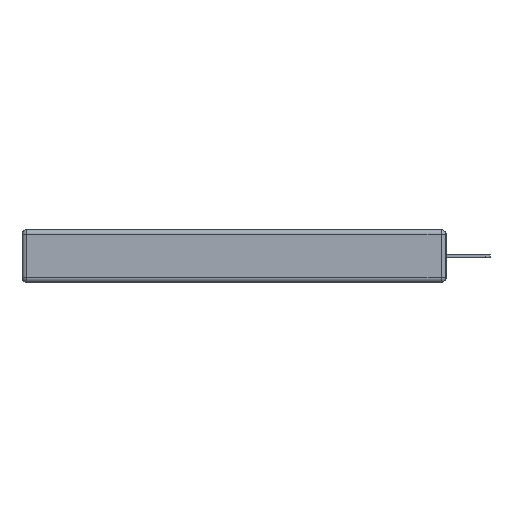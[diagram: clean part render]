
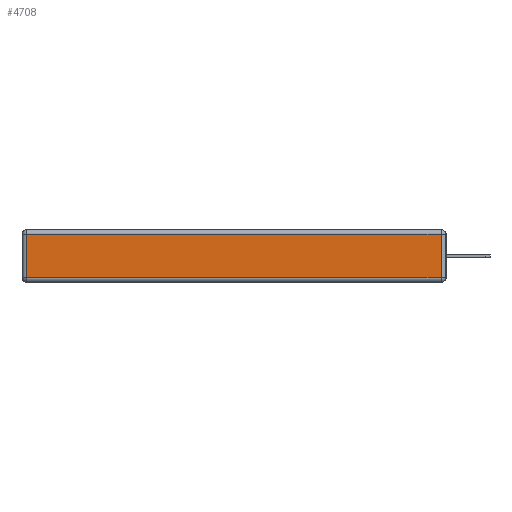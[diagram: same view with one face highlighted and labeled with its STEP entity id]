
A CAD part, left-side view. The second image highlights one B-rep face of the part: STEP entity #4708.
In plain terms, the highlighted planar face has unit normal (-1, 0, 0).
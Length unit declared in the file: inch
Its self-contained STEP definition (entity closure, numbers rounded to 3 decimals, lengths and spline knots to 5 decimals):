
#834 = CARTESIAN_POINT ( 'NONE',  ( 0., 2.72, -0.03 ) ) ;
#927 = EDGE_CURVE ( 'NONE', #22604, #4115, #10498, .T. ) ;
#2394 = CARTESIAN_POINT ( 'NONE',  ( 0., 0., -0.313 ) ) ;
#2729 = VERTEX_POINT ( 'NONE', #834 ) ;
#2935 = VECTOR ( 'NONE', #6644, 39.37008 ) ;
#2946 = CARTESIAN_POINT ( 'NONE',  ( 0., 2.72, -0.313 ) ) ;
#4115 = VERTEX_POINT ( 'NONE', #21625 ) ;
#4242 = EDGE_CURVE ( 'NONE', #6738, #22604, #4624, .T. ) ;
#4624 = LINE ( 'NONE', #2394, #20329 ) ;
#4708 = ADVANCED_FACE ( 'NONE', ( #14742 ), #17619, .T. ) ;
#6498 = ORIENTED_EDGE ( 'NONE', *, *, #17377, .T. ) ;
#6644 = DIRECTION ( 'NONE',  ( 0., 1., 0. ) ) ;
#6738 = VERTEX_POINT ( 'NONE', #2946 ) ;
#6924 = VECTOR ( 'NONE', #21219, 39.37008 ) ;
#7424 = ORIENTED_EDGE ( 'NONE', *, *, #927, .T. ) ;
#8707 = DIRECTION ( 'NONE',  ( 0., -1., 0. ) ) ;
#8857 = LINE ( 'NONE', #8981, #6924 ) ;
#8981 = CARTESIAN_POINT ( 'NONE',  ( 0., 2.72, -0.343 ) ) ;
#9323 = DIRECTION ( 'NONE',  ( 0., 0., 1. ) ) ;
#10401 = VECTOR ( 'NONE', #24332, 39.37008 ) ;
#10498 = LINE ( 'NONE', #16432, #10401 ) ;
#12283 = ORIENTED_EDGE ( 'NONE', *, *, #4242, .T. ) ;
#12835 = CARTESIAN_POINT ( 'NONE',  ( 0., 2.75, -0.03 ) ) ;
#14052 = ORIENTED_EDGE ( 'NONE', *, *, #24858, .T. ) ;
#14742 = FACE_OUTER_BOUND ( 'NONE', #18623, .T. ) ;
#15290 = AXIS2_PLACEMENT_3D ( 'NONE', #15382, #19579, #9323 ) ;
#15382 = CARTESIAN_POINT ( 'NONE',  ( 0., 0., -0.343 ) ) ;
#16432 = CARTESIAN_POINT ( 'NONE',  ( 0., 0.03, -0.343 ) ) ;
#17377 = EDGE_CURVE ( 'NONE', #4115, #2729, #21469, .T. ) ;
#17619 = PLANE ( 'NONE',  #15290 ) ;
#18623 = EDGE_LOOP ( 'NONE', ( #12283, #7424, #6498, #14052 ) ) ;
#19579 = DIRECTION ( 'NONE',  ( -1., 0., 0. ) ) ;
#20329 = VECTOR ( 'NONE', #8707, 39.37008 ) ;
#21219 = DIRECTION ( 'NONE',  ( 0., 0., -1. ) ) ;
#21469 = LINE ( 'NONE', #12835, #2935 ) ;
#21546 = CARTESIAN_POINT ( 'NONE',  ( 0., 0.03, -0.313 ) ) ;
#21625 = CARTESIAN_POINT ( 'NONE',  ( 0., 0.03, -0.03 ) ) ;
#22604 = VERTEX_POINT ( 'NONE', #21546 ) ;
#24332 = DIRECTION ( 'NONE',  ( 0., 0., 1. ) ) ;
#24858 = EDGE_CURVE ( 'NONE', #2729, #6738, #8857, .T. ) ;
